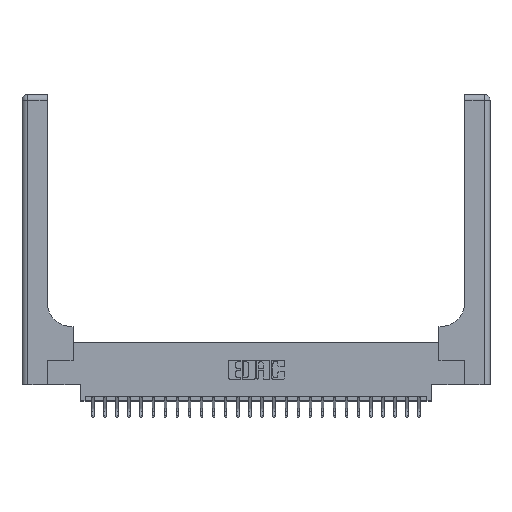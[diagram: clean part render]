
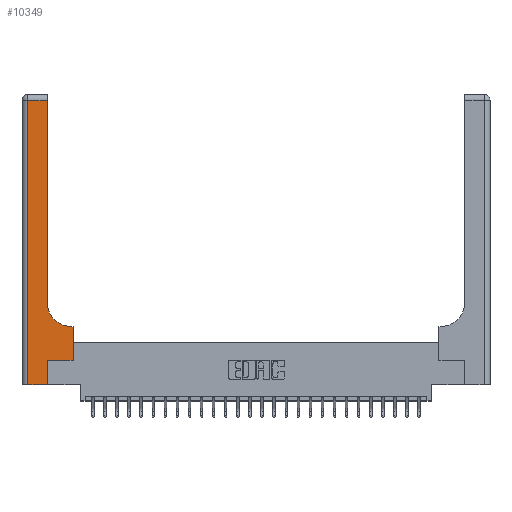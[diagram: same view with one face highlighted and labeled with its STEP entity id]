
A CAD part, top view. The second image highlights one B-rep face of the part: STEP entity #10349.
In plain terms, the highlighted planar face has unit normal (0, 0, 1).
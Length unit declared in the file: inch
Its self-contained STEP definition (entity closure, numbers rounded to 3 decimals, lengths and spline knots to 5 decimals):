
#180 = LINE ( 'NONE', #5036, #3847 ) ;
#726 = VERTEX_POINT ( 'NONE', #11236 ) ;
#1334 = DIRECTION ( 'NONE',  ( 0., 1., 0. ) ) ;
#1358 = CARTESIAN_POINT ( 'NONE',  ( 0.06, 2.94, 0.37 ) ) ;
#1565 = ORIENTED_EDGE ( 'NONE', *, *, #16496, .T. ) ;
#2548 = FACE_OUTER_BOUND ( 'NONE', #20842, .T. ) ;
#2659 = CARTESIAN_POINT ( 'NONE',  ( 0.265, 0., 0.37 ) ) ;
#2739 = VECTOR ( 'NONE', #12069, 39.37008 ) ;
#2815 = CARTESIAN_POINT ( 'NONE',  ( 0., 3., 0.37 ) ) ;
#3081 = LINE ( 'NONE', #19444, #13727 ) ;
#3672 = LINE ( 'NONE', #11759, #16412 ) ;
#3847 = VECTOR ( 'NONE', #10713, 39.37008 ) ;
#4555 = CARTESIAN_POINT ( 'NONE',  ( 0.06, 0., 0.37 ) ) ;
#5036 = CARTESIAN_POINT ( 'NONE',  ( 0.265, 0., 0.37 ) ) ;
#5180 = EDGE_CURVE ( 'NONE', #18413, #726, #180, .T. ) ;
#5281 = AXIS2_PLACEMENT_3D ( 'NONE', #2815, #10449, #22526 ) ;
#5285 = DIRECTION ( 'NONE',  ( 0., 1., 0. ) ) ;
#5452 = LINE ( 'NONE', #9636, #2739 ) ;
#5652 = EDGE_CURVE ( 'NONE', #25459, #18413, #25424, .T. ) ;
#6093 = VECTOR ( 'NONE', #16225, 39.37008 ) ;
#6313 = VECTOR ( 'NONE', #5285, 39.37008 ) ;
#6528 = PLANE ( 'NONE',  #5281 ) ;
#6721 = VERTEX_POINT ( 'NONE', #9563 ) ;
#6794 = EDGE_CURVE ( 'NONE', #17960, #11328, #26044, .T. ) ;
#7104 = CARTESIAN_POINT ( 'NONE',  ( 0.51, 0.6, 0.37 ) ) ;
#7250 = DIRECTION ( 'NONE',  ( 1., 0., 0. ) ) ;
#7464 = DIRECTION ( 'NONE',  ( 0., 0., -1. ) ) ;
#7606 = CARTESIAN_POINT ( 'NONE',  ( 0.51, 0.85, 0.37 ) ) ;
#7870 = CARTESIAN_POINT ( 'NONE',  ( 0., 2.94, 0.37 ) ) ;
#9322 = EDGE_CURVE ( 'NONE', #12365, #17960, #25810, .T. ) ;
#9563 = CARTESIAN_POINT ( 'NONE',  ( 0.528, 0.6, 0.37 ) ) ;
#9578 = ORIENTED_EDGE ( 'NONE', *, *, #5652, .T. ) ;
#9636 = CARTESIAN_POINT ( 'NONE',  ( 0.265, 0.25, 0.37 ) ) ;
#10349 = ADVANCED_FACE ( 'NONE', ( #2548 ), #6528, .F. ) ;
#10449 = DIRECTION ( 'NONE',  ( 0., 0., -1. ) ) ;
#10489 = ORIENTED_EDGE ( 'NONE', *, *, #24386, .T. ) ;
#10713 = DIRECTION ( 'NONE',  ( 0., 1., 0. ) ) ;
#11236 = CARTESIAN_POINT ( 'NONE',  ( 0.265, 0.25, 0.37 ) ) ;
#11328 = VERTEX_POINT ( 'NONE', #1358 ) ;
#11759 = CARTESIAN_POINT ( 'NONE',  ( 0.26, 0.6, 0.37 ) ) ;
#11792 = EDGE_CURVE ( 'NONE', #6721, #21204, #3672, .T. ) ;
#12069 = DIRECTION ( 'NONE',  ( 1., 0., 0. ) ) ;
#12365 = VERTEX_POINT ( 'NONE', #25967 ) ;
#13727 = VECTOR ( 'NONE', #16800, 39.37008 ) ;
#13841 = DIRECTION ( 'NONE',  ( 1., 0., 0. ) ) ;
#14371 = AXIS2_PLACEMENT_3D ( 'NONE', #7606, #7464, #13841 ) ;
#16225 = DIRECTION ( 'NONE',  ( -1., 0., 0. ) ) ;
#16342 = EDGE_CURVE ( 'NONE', #726, #21177, #5452, .T. ) ;
#16412 = VECTOR ( 'NONE', #19803, 39.37008 ) ;
#16496 = EDGE_CURVE ( 'NONE', #11328, #25459, #3081, .T. ) ;
#16525 = ORIENTED_EDGE ( 'NONE', *, *, #16342, .T. ) ;
#16800 = DIRECTION ( 'NONE',  ( 0., -1., 0. ) ) ;
#16817 = CIRCLE ( 'NONE', #14371, 0.25 ) ;
#16870 = ORIENTED_EDGE ( 'NONE', *, *, #9322, .T. ) ;
#17960 = VERTEX_POINT ( 'NONE', #26057 ) ;
#18413 = VERTEX_POINT ( 'NONE', #2659 ) ;
#18584 = VECTOR ( 'NONE', #1334, 39.37008 ) ;
#19444 = CARTESIAN_POINT ( 'NONE',  ( 0.06, 3., 0.37 ) ) ;
#19661 = ORIENTED_EDGE ( 'NONE', *, *, #6794, .T. ) ;
#19803 = DIRECTION ( 'NONE',  ( -1., 0., 0. ) ) ;
#19812 = CARTESIAN_POINT ( 'NONE',  ( 0.528, 0.25, 0.37 ) ) ;
#20842 = EDGE_LOOP ( 'NONE', ( #16870, #19661, #1565, #9578, #23381, #16525, #23079, #24078, #10489 ) ) ;
#21128 = CARTESIAN_POINT ( 'NONE',  ( 0.528, 0.25, 0.37 ) ) ;
#21167 = CARTESIAN_POINT ( 'NONE',  ( 0.26, 3., 0.37 ) ) ;
#21177 = VERTEX_POINT ( 'NONE', #21128 ) ;
#21204 = VERTEX_POINT ( 'NONE', #7104 ) ;
#22526 = DIRECTION ( 'NONE',  ( -1., 0., 0. ) ) ;
#23079 = ORIENTED_EDGE ( 'NONE', *, *, #23118, .T. ) ;
#23118 = EDGE_CURVE ( 'NONE', #21177, #6721, #25302, .T. ) ;
#23381 = ORIENTED_EDGE ( 'NONE', *, *, #5180, .T. ) ;
#23521 = CARTESIAN_POINT ( 'NONE',  ( 0., 0., 0.37 ) ) ;
#24078 = ORIENTED_EDGE ( 'NONE', *, *, #11792, .T. ) ;
#24386 = EDGE_CURVE ( 'NONE', #21204, #12365, #16817, .T. ) ;
#24589 = VECTOR ( 'NONE', #7250, 39.37008 ) ;
#25302 = LINE ( 'NONE', #19812, #6313 ) ;
#25424 = LINE ( 'NONE', #23521, #24589 ) ;
#25459 = VERTEX_POINT ( 'NONE', #4555 ) ;
#25810 = LINE ( 'NONE', #21167, #18584 ) ;
#25967 = CARTESIAN_POINT ( 'NONE',  ( 0.26, 0.85, 0.37 ) ) ;
#26044 = LINE ( 'NONE', #7870, #6093 ) ;
#26057 = CARTESIAN_POINT ( 'NONE',  ( 0.26, 2.94, 0.37 ) ) ;
